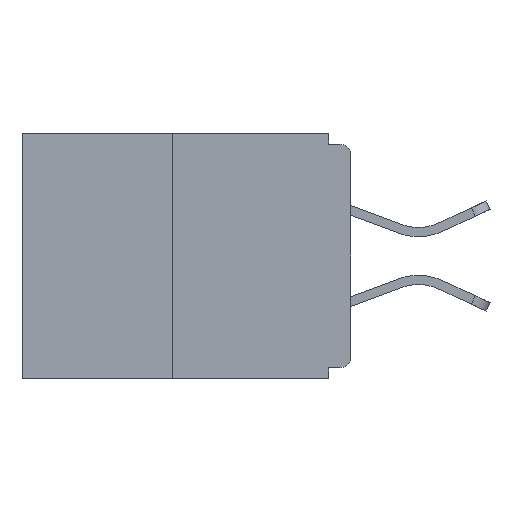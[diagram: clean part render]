
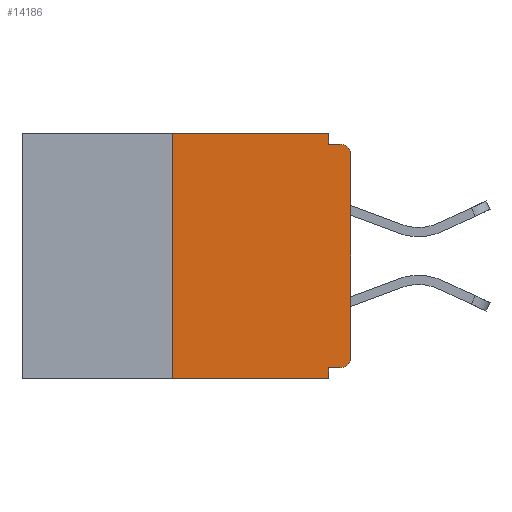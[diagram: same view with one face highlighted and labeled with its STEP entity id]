
A CAD part, left-side view. The second image highlights one B-rep face of the part: STEP entity #14186.
In plain terms, the highlighted planar face has unit normal (-1, 0, 0).
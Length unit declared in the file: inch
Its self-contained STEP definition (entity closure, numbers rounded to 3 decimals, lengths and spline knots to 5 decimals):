
#201 = EDGE_CURVE ( 'NONE', #19971, #9738, #25186, .T. ) ;
#431 = VERTEX_POINT ( 'NONE', #23534 ) ;
#1177 = DIRECTION ( 'NONE',  ( 0., -1., 0. ) ) ;
#1278 = VECTOR ( 'NONE', #6352, 39.37008 ) ;
#1279 = VERTEX_POINT ( 'NONE', #13797 ) ;
#1313 = CARTESIAN_POINT ( 'NONE',  ( 0., 0.031, 0. ) ) ;
#2047 = ORIENTED_EDGE ( 'NONE', *, *, #201, .F. ) ;
#2217 = ORIENTED_EDGE ( 'NONE', *, *, #9491, .F. ) ;
#2358 = CARTESIAN_POINT ( 'NONE',  ( 0., 0.015, -0.328 ) ) ;
#2456 = DIRECTION ( 'NONE',  ( 0., 0., -1. ) ) ;
#2563 = LINE ( 'NONE', #3332, #14083 ) ;
#2953 = EDGE_CURVE ( 'NONE', #3908, #11961, #20693, .T. ) ;
#3312 = FACE_OUTER_BOUND ( 'NONE', #24768, .T. ) ;
#3332 = CARTESIAN_POINT ( 'NONE',  ( 0., 0.031, -0.343 ) ) ;
#3908 = VERTEX_POINT ( 'NONE', #2358 ) ;
#4077 = ORIENTED_EDGE ( 'NONE', *, *, #5191, .F. ) ;
#4444 = CARTESIAN_POINT ( 'NONE',  ( 0., 0., 0. ) ) ;
#4526 = CARTESIAN_POINT ( 'NONE',  ( 0., 0., -0.328 ) ) ;
#4606 = CARTESIAN_POINT ( 'NONE',  ( 0., 0., -0.015 ) ) ;
#4961 = CARTESIAN_POINT ( 'NONE',  ( 0., 0.25, 0. ) ) ;
#5139 = EDGE_CURVE ( 'NONE', #11961, #10088, #2563, .T. ) ;
#5178 = CARTESIAN_POINT ( 'NONE',  ( 0., 0.031, -0.343 ) ) ;
#5191 = EDGE_CURVE ( 'NONE', #9738, #431, #6578, .T. ) ;
#6233 = CARTESIAN_POINT ( 'NONE',  ( 0., 0.25, 0. ) ) ;
#6296 = CARTESIAN_POINT ( 'NONE',  ( 0., 0.015, -0.015 ) ) ;
#6352 = DIRECTION ( 'NONE',  ( 0., 0., 1. ) ) ;
#6381 = AXIS2_PLACEMENT_3D ( 'NONE', #8202, #14396, #2456 ) ;
#6422 = ORIENTED_EDGE ( 'NONE', *, *, #17183, .T. ) ;
#6578 = LINE ( 'NONE', #21636, #11921 ) ;
#6977 = VERTEX_POINT ( 'NONE', #6296 ) ;
#7324 = LINE ( 'NONE', #4606, #18832 ) ;
#8202 = CARTESIAN_POINT ( 'NONE',  ( 0., 0.015, -0.313 ) ) ;
#8762 = LINE ( 'NONE', #4444, #1278 ) ;
#9410 = VECTOR ( 'NONE', #10976, 39.37008 ) ;
#9491 = EDGE_CURVE ( 'NONE', #431, #6977, #7324, .T. ) ;
#9622 = CARTESIAN_POINT ( 'NONE',  ( 0., 0.015, -0.03 ) ) ;
#9738 = VERTEX_POINT ( 'NONE', #1313 ) ;
#10088 = VERTEX_POINT ( 'NONE', #5178 ) ;
#10092 = AXIS2_PLACEMENT_3D ( 'NONE', #9622, #23970, #25760 ) ;
#10348 = ORIENTED_EDGE ( 'NONE', *, *, #15415, .T. ) ;
#10857 = LINE ( 'NONE', #17039, #13997 ) ;
#10976 = DIRECTION ( 'NONE',  ( 0., 0., 1. ) ) ;
#11302 = DIRECTION ( 'NONE',  ( 0., 0., -1. ) ) ;
#11542 = ORIENTED_EDGE ( 'NONE', *, *, #2953, .F. ) ;
#11921 = VECTOR ( 'NONE', #21365, 39.37008 ) ;
#11961 = VERTEX_POINT ( 'NONE', #19288 ) ;
#12909 = DIRECTION ( 'NONE',  ( 0., -1., 0. ) ) ;
#13713 = VECTOR ( 'NONE', #12909, 39.37008 ) ;
#13797 = CARTESIAN_POINT ( 'NONE',  ( 0., 0.25, -0.343 ) ) ;
#13997 = VECTOR ( 'NONE', #1177, 39.37008 ) ;
#14083 = VECTOR ( 'NONE', #22831, 39.37008 ) ;
#14186 = ADVANCED_FACE ( 'NONE', ( #3312 ), #20787, .F. ) ;
#14396 = DIRECTION ( 'NONE',  ( -1., 0., 0. ) ) ;
#15311 = ORIENTED_EDGE ( 'NONE', *, *, #21498, .T. ) ;
#15415 = EDGE_CURVE ( 'NONE', #3908, #19177, #25684, .T. ) ;
#16422 = EDGE_CURVE ( 'NONE', #1279, #19971, #22204, .T. ) ;
#16573 = ORIENTED_EDGE ( 'NONE', *, *, #16422, .F. ) ;
#16828 = CARTESIAN_POINT ( 'NONE',  ( 0., 0.46, 0. ) ) ;
#16890 = CIRCLE ( 'NONE', #10092, 0.015 ) ;
#17039 = CARTESIAN_POINT ( 'NONE',  ( 0., 0.46, -0.343 ) ) ;
#17183 = EDGE_CURVE ( 'NONE', #17234, #6977, #16890, .T. ) ;
#17234 = VERTEX_POINT ( 'NONE', #19549 ) ;
#17273 = VECTOR ( 'NONE', #18123, 39.37008 ) ;
#18123 = DIRECTION ( 'NONE',  ( 0., 1., 0. ) ) ;
#18621 = CARTESIAN_POINT ( 'NONE',  ( 0., 0., -0.313 ) ) ;
#18779 = CARTESIAN_POINT ( 'NONE',  ( 0., 0.46, 0. ) ) ;
#18832 = VECTOR ( 'NONE', #20452, 39.37008 ) ;
#19177 = VERTEX_POINT ( 'NONE', #18621 ) ;
#19288 = CARTESIAN_POINT ( 'NONE',  ( 0., 0.031, -0.328 ) ) ;
#19485 = EDGE_CURVE ( 'NONE', #19177, #17234, #8762, .T. ) ;
#19549 = CARTESIAN_POINT ( 'NONE',  ( 0., 0., -0.03 ) ) ;
#19971 = VERTEX_POINT ( 'NONE', #6233 ) ;
#20452 = DIRECTION ( 'NONE',  ( 0., -1., 0. ) ) ;
#20693 = LINE ( 'NONE', #4526, #17273 ) ;
#20787 = PLANE ( 'NONE',  #21223 ) ;
#21223 = AXIS2_PLACEMENT_3D ( 'NONE', #18779, #23281, #11302 ) ;
#21365 = DIRECTION ( 'NONE',  ( 0., 0., -1. ) ) ;
#21498 = EDGE_CURVE ( 'NONE', #1279, #10088, #10857, .T. ) ;
#21636 = CARTESIAN_POINT ( 'NONE',  ( 0., 0.031, 0. ) ) ;
#22204 = LINE ( 'NONE', #4961, #9410 ) ;
#22831 = DIRECTION ( 'NONE',  ( 0., 0., -1. ) ) ;
#23281 = DIRECTION ( 'NONE',  ( 1., 0., 0. ) ) ;
#23534 = CARTESIAN_POINT ( 'NONE',  ( 0., 0.031, -0.015 ) ) ;
#23548 = ORIENTED_EDGE ( 'NONE', *, *, #19485, .T. ) ;
#23970 = DIRECTION ( 'NONE',  ( -1., 0., 0. ) ) ;
#24159 = ORIENTED_EDGE ( 'NONE', *, *, #5139, .F. ) ;
#24768 = EDGE_LOOP ( 'NONE', ( #2047, #16573, #15311, #24159, #11542, #10348, #23548, #6422, #2217, #4077 ) ) ;
#25186 = LINE ( 'NONE', #16828, #13713 ) ;
#25684 = CIRCLE ( 'NONE', #6381, 0.015 ) ;
#25760 = DIRECTION ( 'NONE',  ( 0., 0., -1. ) ) ;
